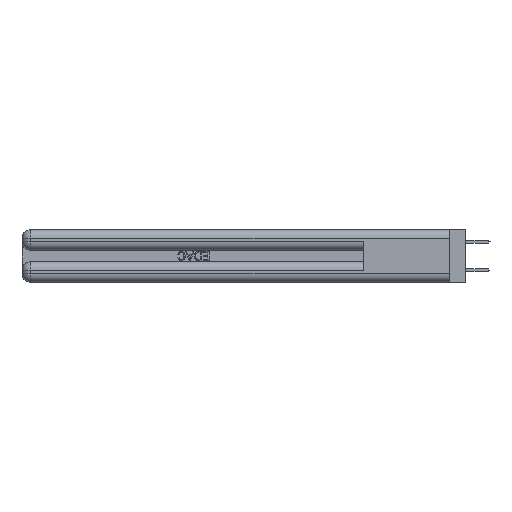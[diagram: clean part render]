
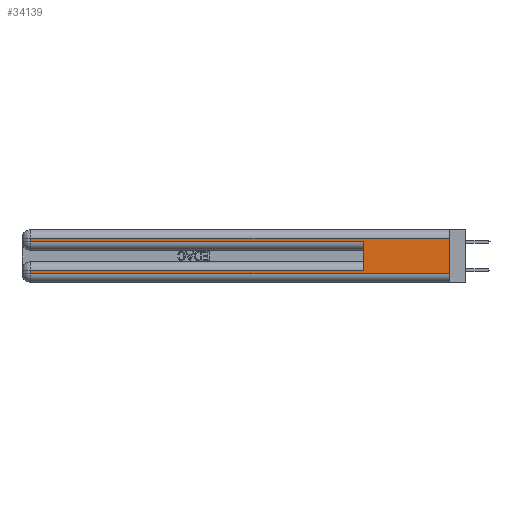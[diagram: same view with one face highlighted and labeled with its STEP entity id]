
A CAD part, left-side view. The second image highlights one B-rep face of the part: STEP entity #34139.
In plain terms, the highlighted planar face has unit normal (-1, 0, 0).
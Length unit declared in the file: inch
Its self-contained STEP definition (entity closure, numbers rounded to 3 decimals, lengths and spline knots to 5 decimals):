
#665 = VERTEX_POINT ( 'NONE', #37119 ) ;
#860 = ORIENTED_EDGE ( 'NONE', *, *, #33816, .T. ) ;
#1175 = CARTESIAN_POINT ( 'NONE',  ( 0., 2.94, 0.06 ) ) ;
#1313 = VERTEX_POINT ( 'NONE', #30603 ) ;
#1537 = VECTOR ( 'NONE', #19467, 39.37008 ) ;
#3417 = DIRECTION ( 'NONE',  ( 0., 0., -1. ) ) ;
#4099 = DIRECTION ( 'NONE',  ( 0., 0., -1. ) ) ;
#4804 = LINE ( 'NONE', #5088, #1537 ) ;
#5088 = CARTESIAN_POINT ( 'NONE',  ( 0., 0., 0.06 ) ) ;
#5862 = CARTESIAN_POINT ( 'NONE',  ( 0., 2.94, 0.085 ) ) ;
#6892 = ORIENTED_EDGE ( 'NONE', *, *, #15254, .T. ) ;
#7588 = PLANE ( 'NONE',  #36650 ) ;
#8662 = CARTESIAN_POINT ( 'NONE',  ( 0., 0.6, 0.145 ) ) ;
#9431 = LINE ( 'NONE', #16926, #29045 ) ;
#10051 = ORIENTED_EDGE ( 'NONE', *, *, #33650, .F. ) ;
#10081 = VECTOR ( 'NONE', #28923, 39.37008 ) ;
#10331 = VERTEX_POINT ( 'NONE', #35084 ) ;
#10401 = VERTEX_POINT ( 'NONE', #1175 ) ;
#10629 = LINE ( 'NONE', #20524, #12435 ) ;
#10889 = VERTEX_POINT ( 'NONE', #11473 ) ;
#10954 = LINE ( 'NONE', #27221, #35130 ) ;
#11473 = CARTESIAN_POINT ( 'NONE',  ( 0., 2.94, 0.31 ) ) ;
#11600 = FACE_OUTER_BOUND ( 'NONE', #15046, .T. ) ;
#11800 = DIRECTION ( 'NONE',  ( 0., 1., 0. ) ) ;
#12277 = EDGE_CURVE ( 'NONE', #1313, #665, #10954, .T. ) ;
#12435 = VECTOR ( 'NONE', #3417, 39.37008 ) ;
#12811 = CARTESIAN_POINT ( 'NONE',  ( 0., 0.6, 0.085 ) ) ;
#13013 = ORIENTED_EDGE ( 'NONE', *, *, #20978, .F. ) ;
#14276 = EDGE_CURVE ( 'NONE', #25667, #36115, #9431, .T. ) ;
#15046 = EDGE_LOOP ( 'NONE', ( #13013, #860, #6892, #31212, #10051, #35034, #16491, #30768 ) ) ;
#15254 = EDGE_CURVE ( 'NONE', #10889, #1313, #15718, .T. ) ;
#15718 = LINE ( 'NONE', #33083, #21170 ) ;
#16491 = ORIENTED_EDGE ( 'NONE', *, *, #17303, .T. ) ;
#16926 = CARTESIAN_POINT ( 'NONE',  ( 0., 0., 0.085 ) ) ;
#17303 = EDGE_CURVE ( 'NONE', #36115, #10401, #21915, .T. ) ;
#19292 = CARTESIAN_POINT ( 'NONE',  ( 0., 0., 0.37 ) ) ;
#19467 = DIRECTION ( 'NONE',  ( 0., -1., 0. ) ) ;
#19820 = VECTOR ( 'NONE', #20702, 39.37008 ) ;
#20524 = CARTESIAN_POINT ( 'NONE',  ( 0., 0., 0.37 ) ) ;
#20702 = DIRECTION ( 'NONE',  ( 0., 1., 0. ) ) ;
#20978 = EDGE_CURVE ( 'NONE', #10331, #21502, #10629, .T. ) ;
#21055 = CARTESIAN_POINT ( 'NONE',  ( 0., 0., 0.06 ) ) ;
#21170 = VECTOR ( 'NONE', #24410, 39.37008 ) ;
#21502 = VERTEX_POINT ( 'NONE', #21055 ) ;
#21915 = LINE ( 'NONE', #23070, #10081 ) ;
#23027 = DIRECTION ( 'NONE',  ( 0., 0., 1. ) ) ;
#23070 = CARTESIAN_POINT ( 'NONE',  ( 0., 2.94, 0.37 ) ) ;
#24410 = DIRECTION ( 'NONE',  ( 0., 0., -1. ) ) ;
#24687 = DIRECTION ( 'NONE',  ( 0., -1., 0. ) ) ;
#25667 = VERTEX_POINT ( 'NONE', #12811 ) ;
#27221 = CARTESIAN_POINT ( 'NONE',  ( 0., 0., 0.285 ) ) ;
#27639 = DIRECTION ( 'NONE',  ( 1., 0., 0. ) ) ;
#28923 = DIRECTION ( 'NONE',  ( 0., 0., -1. ) ) ;
#29045 = VECTOR ( 'NONE', #11800, 39.37008 ) ;
#29369 = CARTESIAN_POINT ( 'NONE',  ( 0., 0., 0.31 ) ) ;
#29807 = LINE ( 'NONE', #8662, #37178 ) ;
#30603 = CARTESIAN_POINT ( 'NONE',  ( 0., 2.94, 0.285 ) ) ;
#30768 = ORIENTED_EDGE ( 'NONE', *, *, #33543, .T. ) ;
#31212 = ORIENTED_EDGE ( 'NONE', *, *, #12277, .T. ) ;
#33083 = CARTESIAN_POINT ( 'NONE',  ( 0., 2.94, 0.37 ) ) ;
#33543 = EDGE_CURVE ( 'NONE', #10401, #21502, #4804, .T. ) ;
#33650 = EDGE_CURVE ( 'NONE', #25667, #665, #29807, .T. ) ;
#33816 = EDGE_CURVE ( 'NONE', #10331, #10889, #34417, .T. ) ;
#34139 = ADVANCED_FACE ( 'NONE', ( #11600 ), #7588, .F. ) ;
#34417 = LINE ( 'NONE', #29369, #19820 ) ;
#35034 = ORIENTED_EDGE ( 'NONE', *, *, #14276, .T. ) ;
#35084 = CARTESIAN_POINT ( 'NONE',  ( 0., 0., 0.31 ) ) ;
#35130 = VECTOR ( 'NONE', #24687, 39.37008 ) ;
#36115 = VERTEX_POINT ( 'NONE', #5862 ) ;
#36650 = AXIS2_PLACEMENT_3D ( 'NONE', #19292, #27639, #4099 ) ;
#37119 = CARTESIAN_POINT ( 'NONE',  ( 0., 0.6, 0.285 ) ) ;
#37178 = VECTOR ( 'NONE', #23027, 39.37008 ) ;
